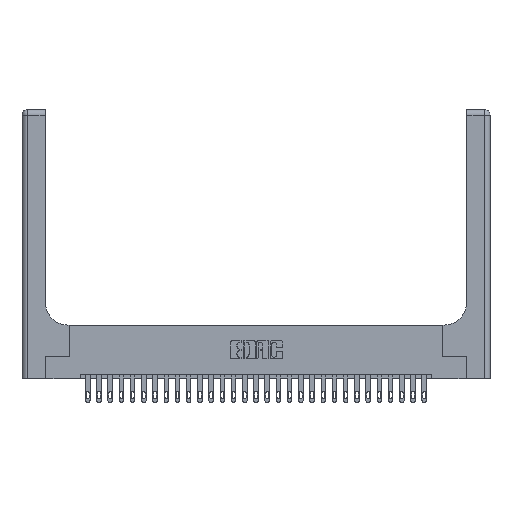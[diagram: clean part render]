
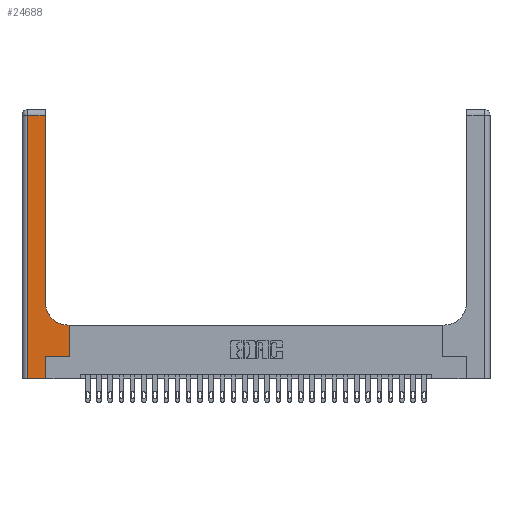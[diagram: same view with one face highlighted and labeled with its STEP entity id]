
A CAD part, top view. The second image highlights one B-rep face of the part: STEP entity #24688.
In plain terms, the highlighted planar face has unit normal (0, 0, 1).
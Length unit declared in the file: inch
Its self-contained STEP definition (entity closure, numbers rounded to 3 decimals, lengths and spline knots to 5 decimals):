
#640 = DIRECTION ( 'NONE',  ( 0., 1., 0. ) ) ;
#775 = VERTEX_POINT ( 'NONE', #21087 ) ;
#1135 = CARTESIAN_POINT ( 'NONE',  ( 0., 2.94, 0.37 ) ) ;
#1439 = LINE ( 'NONE', #7779, #3542 ) ;
#1613 = CARTESIAN_POINT ( 'NONE',  ( 0.06, 3., 0.37 ) ) ;
#1912 = DIRECTION ( 'NONE',  ( 0., 0., -1. ) ) ;
#2944 = ORIENTED_EDGE ( 'NONE', *, *, #26801, .T. ) ;
#3524 = EDGE_CURVE ( 'NONE', #18158, #15450, #12301, .T. ) ;
#3542 = VECTOR ( 'NONE', #11387, 39.37008 ) ;
#3944 = EDGE_CURVE ( 'NONE', #15450, #775, #22590, .T. ) ;
#4177 = LINE ( 'NONE', #25605, #27152 ) ;
#4747 = DIRECTION ( 'NONE',  ( 1., 0., 0. ) ) ;
#4777 = VECTOR ( 'NONE', #640, 39.37008 ) ;
#4793 = CARTESIAN_POINT ( 'NONE',  ( 0.528, 0.6, 0.37 ) ) ;
#4874 = AXIS2_PLACEMENT_3D ( 'NONE', #5879, #22994, #8222 ) ;
#5072 = EDGE_CURVE ( 'NONE', #14300, #10057, #5273, .T. ) ;
#5273 = LINE ( 'NONE', #1135, #9586 ) ;
#5879 = CARTESIAN_POINT ( 'NONE',  ( 0., 3., 0.37 ) ) ;
#6078 = CARTESIAN_POINT ( 'NONE',  ( 0.26, 0.6, 0.37 ) ) ;
#6639 = EDGE_CURVE ( 'NONE', #17157, #14962, #4177, .T. ) ;
#6654 = CARTESIAN_POINT ( 'NONE',  ( 0.06, 0., 0.37 ) ) ;
#7167 = AXIS2_PLACEMENT_3D ( 'NONE', #11998, #1912, #18891 ) ;
#7747 = DIRECTION ( 'NONE',  ( -1., 0., 0. ) ) ;
#7779 = CARTESIAN_POINT ( 'NONE',  ( 0.265, 0.25, 0.37 ) ) ;
#8222 = DIRECTION ( 'NONE',  ( -1., 0., 0. ) ) ;
#8339 = CARTESIAN_POINT ( 'NONE',  ( 0.51, 0.6, 0.37 ) ) ;
#8429 = DIRECTION ( 'NONE',  ( -1., 0., 0. ) ) ;
#8646 = CARTESIAN_POINT ( 'NONE',  ( 0.265, 0., 0.37 ) ) ;
#9586 = VECTOR ( 'NONE', #7747, 39.37008 ) ;
#10057 = VERTEX_POINT ( 'NONE', #24602 ) ;
#10403 = ORIENTED_EDGE ( 'NONE', *, *, #3944, .T. ) ;
#11102 = VECTOR ( 'NONE', #25558, 39.37008 ) ;
#11387 = DIRECTION ( 'NONE',  ( 1., 0., 0. ) ) ;
#11518 = LINE ( 'NONE', #19674, #23283 ) ;
#11998 = CARTESIAN_POINT ( 'NONE',  ( 0.51, 0.85, 0.37 ) ) ;
#12117 = VERTEX_POINT ( 'NONE', #14907 ) ;
#12233 = LINE ( 'NONE', #1613, #12655 ) ;
#12301 = LINE ( 'NONE', #6078, #24394 ) ;
#12557 = LINE ( 'NONE', #23048, #11102 ) ;
#12655 = VECTOR ( 'NONE', #20660, 39.37008 ) ;
#13397 = EDGE_CURVE ( 'NONE', #10057, #17157, #12233, .T. ) ;
#13592 = DIRECTION ( 'NONE',  ( 0., 1., 0. ) ) ;
#14300 = VERTEX_POINT ( 'NONE', #14344 ) ;
#14344 = CARTESIAN_POINT ( 'NONE',  ( 0.26, 2.94, 0.37 ) ) ;
#14521 = ORIENTED_EDGE ( 'NONE', *, *, #22028, .T. ) ;
#14804 = VERTEX_POINT ( 'NONE', #27166 ) ;
#14907 = CARTESIAN_POINT ( 'NONE',  ( 0.528, 0.25, 0.37 ) ) ;
#14962 = VERTEX_POINT ( 'NONE', #8646 ) ;
#15396 = CARTESIAN_POINT ( 'NONE',  ( 0.26, 3., 0.37 ) ) ;
#15450 = VERTEX_POINT ( 'NONE', #8339 ) ;
#16784 = FACE_OUTER_BOUND ( 'NONE', #26686, .T. ) ;
#17157 = VERTEX_POINT ( 'NONE', #6654 ) ;
#18158 = VERTEX_POINT ( 'NONE', #4793 ) ;
#18891 = DIRECTION ( 'NONE',  ( 1., 0., 0. ) ) ;
#19030 = ORIENTED_EDGE ( 'NONE', *, *, #5072, .T. ) ;
#19257 = ORIENTED_EDGE ( 'NONE', *, *, #25101, .T. ) ;
#19674 = CARTESIAN_POINT ( 'NONE',  ( 0.265, 0., 0.37 ) ) ;
#20660 = DIRECTION ( 'NONE',  ( 0., -1., 0. ) ) ;
#21087 = CARTESIAN_POINT ( 'NONE',  ( 0.26, 0.85, 0.37 ) ) ;
#21869 = LINE ( 'NONE', #15396, #4777 ) ;
#21941 = EDGE_CURVE ( 'NONE', #775, #14300, #21869, .T. ) ;
#22028 = EDGE_CURVE ( 'NONE', #14962, #14804, #11518, .T. ) ;
#22097 = ORIENTED_EDGE ( 'NONE', *, *, #13397, .T. ) ;
#22590 = CIRCLE ( 'NONE', #7167, 0.25 ) ;
#22994 = DIRECTION ( 'NONE',  ( 0., 0., -1. ) ) ;
#23048 = CARTESIAN_POINT ( 'NONE',  ( 0.528, 0.25, 0.37 ) ) ;
#23283 = VECTOR ( 'NONE', #13592, 39.37008 ) ;
#24394 = VECTOR ( 'NONE', #8429, 39.37008 ) ;
#24602 = CARTESIAN_POINT ( 'NONE',  ( 0.06, 2.94, 0.37 ) ) ;
#24688 = ADVANCED_FACE ( 'NONE', ( #16784 ), #24940, .F. ) ;
#24767 = ORIENTED_EDGE ( 'NONE', *, *, #3524, .T. ) ;
#24940 = PLANE ( 'NONE',  #4874 ) ;
#25101 = EDGE_CURVE ( 'NONE', #14804, #12117, #1439, .T. ) ;
#25558 = DIRECTION ( 'NONE',  ( 0., 1., 0. ) ) ;
#25605 = CARTESIAN_POINT ( 'NONE',  ( 0., 0., 0.37 ) ) ;
#25852 = ORIENTED_EDGE ( 'NONE', *, *, #21941, .T. ) ;
#26096 = ORIENTED_EDGE ( 'NONE', *, *, #6639, .T. ) ;
#26686 = EDGE_LOOP ( 'NONE', ( #25852, #19030, #22097, #26096, #14521, #19257, #2944, #24767, #10403 ) ) ;
#26801 = EDGE_CURVE ( 'NONE', #12117, #18158, #12557, .T. ) ;
#27152 = VECTOR ( 'NONE', #4747, 39.37008 ) ;
#27166 = CARTESIAN_POINT ( 'NONE',  ( 0.265, 0.25, 0.37 ) ) ;
